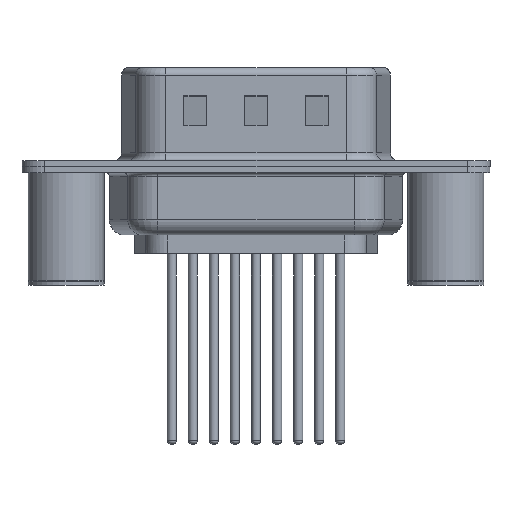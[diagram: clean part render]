
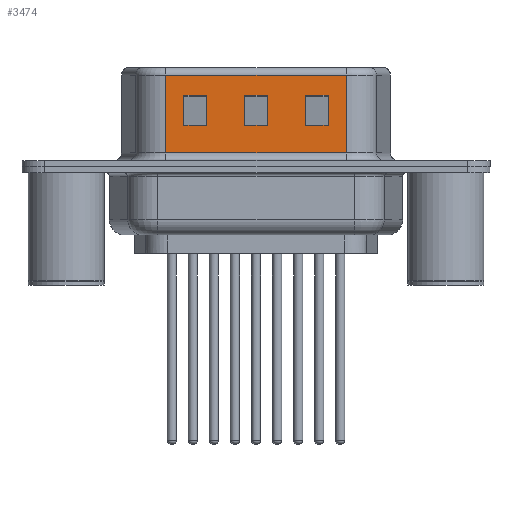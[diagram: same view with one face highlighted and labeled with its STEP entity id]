
A CAD part, front view. The second image highlights one B-rep face of the part: STEP entity #3474.
In plain terms, the highlighted planar face has unit normal (0, -1, 0).
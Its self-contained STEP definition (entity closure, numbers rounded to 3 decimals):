
#218 = CARTESIAN_POINT ( 'NONE',  ( 7.75, -4.55, 2.705 ) ) ;
#254 = CARTESIAN_POINT ( 'NONE',  ( 14.451, -4.55, 2.705 ) ) ;
#311 = DIRECTION ( 'NONE',  ( -1., 0., 0. ) ) ;
#480 = CARTESIAN_POINT ( 'NONE',  ( 22.451, -4.55, 2.705 ) ) ;
#491 = CARTESIAN_POINT ( 'NONE',  ( 11.75, -4.55, 6.52 ) ) ;
#503 = CARTESIAN_POINT ( 'NONE',  ( 18.451, -4.55, 0.9 ) ) ;
#578 = CARTESIAN_POINT ( 'NONE',  ( 9.25, -4.55, 4.705 ) ) ;
#632 = CARTESIAN_POINT ( 'NONE',  ( 6.549, -4.55, 6.02 ) ) ;
#977 = VERTEX_POINT ( 'NONE', #578 ) ;
#1169 = CARTESIAN_POINT ( 'NONE',  ( 18.451, -4.55, 4.705 ) ) ;
#1282 = VERTEX_POINT ( 'NONE', #12414 ) ;
#1305 = LINE ( 'NONE', #480, #1506 ) ;
#1433 = CARTESIAN_POINT ( 'NONE',  ( 17.25, -4.55, 2.705 ) ) ;
#1506 = VECTOR ( 'NONE', #10874, 1000. ) ;
#1622 = EDGE_CURVE ( 'NONE', #1282, #977, #7568, .T. ) ;
#1678 = VERTEX_POINT ( 'NONE', #4030 ) ;
#1951 = CARTESIAN_POINT ( 'NONE',  ( 14.451, -4.55, 4.705 ) ) ;
#2179 = ORIENTED_EDGE ( 'NONE', *, *, #2332, .F. ) ;
#2308 = DIRECTION ( 'NONE',  ( 0., 0., 1. ) ) ;
#2332 = EDGE_CURVE ( 'NONE', #5560, #8779, #4738, .T. ) ;
#2356 = EDGE_CURVE ( 'NONE', #13683, #6903, #7967, .T. ) ;
#2851 = CARTESIAN_POINT ( 'NONE',  ( 15.75, -4.55, 6.52 ) ) ;
#2897 = VERTEX_POINT ( 'NONE', #1433 ) ;
#3019 = CARTESIAN_POINT ( 'NONE',  ( 7.75, -4.55, 6.52 ) ) ;
#3036 = ORIENTED_EDGE ( 'NONE', *, *, #8188, .T. ) ;
#3043 = VERTEX_POINT ( 'NONE', #6137 ) ;
#3084 = DIRECTION ( 'NONE',  ( 0., 0., -1. ) ) ;
#3296 = CARTESIAN_POINT ( 'NONE',  ( 18.451, -4.55, 0.9 ) ) ;
#3410 = ORIENTED_EDGE ( 'NONE', *, *, #10835, .T. ) ;
#3474 = ADVANCED_FACE ( 'NONE', ( #7846, #12487, #13536, #14818 ), #11289, .F. ) ;
#3587 = DIRECTION ( 'NONE',  ( 0., 0., -1. ) ) ;
#3903 = VECTOR ( 'NONE', #8540, 1000. ) ;
#4028 = VECTOR ( 'NONE', #6989, 1000. ) ;
#4030 = CARTESIAN_POINT ( 'NONE',  ( 6.549, -4.55, 0.9 ) ) ;
#4054 = EDGE_CURVE ( 'NONE', #2897, #3043, #1305, .T. ) ;
#4115 = CARTESIAN_POINT ( 'NONE',  ( 9.25, -4.55, 6.52 ) ) ;
#4258 = LINE ( 'NONE', #3296, #7991 ) ;
#4315 = VERTEX_POINT ( 'NONE', #9978 ) ;
#4575 = EDGE_CURVE ( 'NONE', #14116, #4315, #5269, .T. ) ;
#4643 = EDGE_CURVE ( 'NONE', #6903, #1282, #14329, .T. ) ;
#4707 = CARTESIAN_POINT ( 'NONE',  ( 17.25, -4.55, 6.52 ) ) ;
#4738 = LINE ( 'NONE', #6979, #11361 ) ;
#4763 = ORIENTED_EDGE ( 'NONE', *, *, #12984, .T. ) ;
#4870 = DIRECTION ( 'NONE',  ( 1., 0., 0. ) ) ;
#4931 = CARTESIAN_POINT ( 'NONE',  ( 18.451, -4.55, 6.02 ) ) ;
#4947 = LINE ( 'NONE', #6851, #12132 ) ;
#4975 = LINE ( 'NONE', #491, #10548 ) ;
#5015 = EDGE_LOOP ( 'NONE', ( #3036, #10046, #6548, #5702 ) ) ;
#5024 = EDGE_CURVE ( 'NONE', #3043, #6532, #7494, .T. ) ;
#5044 = VECTOR ( 'NONE', #3084, 1000. ) ;
#5077 = EDGE_CURVE ( 'NONE', #4315, #6470, #13031, .T. ) ;
#5103 = VECTOR ( 'NONE', #6162, 1000. ) ;
#5244 = CARTESIAN_POINT ( 'NONE',  ( 11.75, -4.55, 2.705 ) ) ;
#5247 = CARTESIAN_POINT ( 'NONE',  ( 18.451, -4.55, 2.705 ) ) ;
#5269 = LINE ( 'NONE', #10876, #7737 ) ;
#5286 = VECTOR ( 'NONE', #9159, 1000. ) ;
#5560 = VERTEX_POINT ( 'NONE', #4931 ) ;
#5702 = ORIENTED_EDGE ( 'NONE', *, *, #9033, .T. ) ;
#5853 = LINE ( 'NONE', #8173, #14726 ) ;
#6130 = EDGE_LOOP ( 'NONE', ( #2179, #13616, #13368, #8564 ) ) ;
#6137 = CARTESIAN_POINT ( 'NONE',  ( 15.75, -4.55, 2.705 ) ) ;
#6162 = DIRECTION ( 'NONE',  ( 0., 0., 1. ) ) ;
#6470 = VERTEX_POINT ( 'NONE', #5244 ) ;
#6532 = VERTEX_POINT ( 'NONE', #7413 ) ;
#6548 = ORIENTED_EDGE ( 'NONE', *, *, #5024, .T. ) ;
#6584 = VECTOR ( 'NONE', #12469, 1000. ) ;
#6648 = EDGE_CURVE ( 'NONE', #1678, #8779, #4258, .T. ) ;
#6851 = CARTESIAN_POINT ( 'NONE',  ( 22.451, -4.55, 4.705 ) ) ;
#6903 = VERTEX_POINT ( 'NONE', #218 ) ;
#6979 = CARTESIAN_POINT ( 'NONE',  ( 18.451, -4.55, 6.52 ) ) ;
#6989 = DIRECTION ( 'NONE',  ( 1., 0., 0. ) ) ;
#7223 = VECTOR ( 'NONE', #9804, 1000. ) ;
#7413 = CARTESIAN_POINT ( 'NONE',  ( 15.75, -4.55, 4.705 ) ) ;
#7473 = ORIENTED_EDGE ( 'NONE', *, *, #4643, .T. ) ;
#7494 = LINE ( 'NONE', #2851, #8460 ) ;
#7542 = CARTESIAN_POINT ( 'NONE',  ( 11.75, -4.55, 4.705 ) ) ;
#7568 = LINE ( 'NONE', #1951, #7223 ) ;
#7737 = VECTOR ( 'NONE', #8709, 1000. ) ;
#7845 = EDGE_CURVE ( 'NONE', #5560, #10954, #5853, .T. ) ;
#7846 = FACE_BOUND ( 'NONE', #14136, .T. ) ;
#7905 = LINE ( 'NONE', #1169, #4028 ) ;
#7967 = LINE ( 'NONE', #254, #6584 ) ;
#7991 = VECTOR ( 'NONE', #8911, 1000. ) ;
#8173 = CARTESIAN_POINT ( 'NONE',  ( 18.451, -4.55, 6.02 ) ) ;
#8188 = EDGE_CURVE ( 'NONE', #12977, #2897, #11604, .T. ) ;
#8460 = VECTOR ( 'NONE', #10931, 1000. ) ;
#8540 = DIRECTION ( 'NONE',  ( -1., 0., 0. ) ) ;
#8564 = ORIENTED_EDGE ( 'NONE', *, *, #6648, .T. ) ;
#8709 = DIRECTION ( 'NONE',  ( 0., 0., -1. ) ) ;
#8731 = ORIENTED_EDGE ( 'NONE', *, *, #2356, .T. ) ;
#8779 = VERTEX_POINT ( 'NONE', #503 ) ;
#8911 = DIRECTION ( 'NONE',  ( 1., 0., 0. ) ) ;
#8938 = VERTEX_POINT ( 'NONE', #7542 ) ;
#9033 = EDGE_CURVE ( 'NONE', #6532, #12977, #4947, .T. ) ;
#9159 = DIRECTION ( 'NONE',  ( 0., 0., -1. ) ) ;
#9163 = ORIENTED_EDGE ( 'NONE', *, *, #4575, .T. ) ;
#9224 = VECTOR ( 'NONE', #3587, 1000. ) ;
#9248 = ORIENTED_EDGE ( 'NONE', *, *, #1622, .T. ) ;
#9375 = EDGE_LOOP ( 'NONE', ( #3410, #9163, #9984, #11782 ) ) ;
#9768 = CARTESIAN_POINT ( 'NONE',  ( 9.25, -4.55, 2.705 ) ) ;
#9804 = DIRECTION ( 'NONE',  ( 1., 0., 0. ) ) ;
#9978 = CARTESIAN_POINT ( 'NONE',  ( 13.25, -4.55, 2.705 ) ) ;
#9984 = ORIENTED_EDGE ( 'NONE', *, *, #5077, .T. ) ;
#10046 = ORIENTED_EDGE ( 'NONE', *, *, #4054, .T. ) ;
#10548 = VECTOR ( 'NONE', #10737, 1000. ) ;
#10737 = DIRECTION ( 'NONE',  ( 0., 0., 1. ) ) ;
#10835 = EDGE_CURVE ( 'NONE', #8938, #14116, #7905, .T. ) ;
#10874 = DIRECTION ( 'NONE',  ( -1., 0., 0. ) ) ;
#10876 = CARTESIAN_POINT ( 'NONE',  ( 13.25, -4.55, 6.52 ) ) ;
#10931 = DIRECTION ( 'NONE',  ( 0., 0., 1. ) ) ;
#10954 = VERTEX_POINT ( 'NONE', #632 ) ;
#11289 = PLANE ( 'NONE',  #13202 ) ;
#11361 = VECTOR ( 'NONE', #11556, 1000. ) ;
#11556 = DIRECTION ( 'NONE',  ( 0., 0., -1. ) ) ;
#11604 = LINE ( 'NONE', #4707, #9224 ) ;
#11782 = ORIENTED_EDGE ( 'NONE', *, *, #13592, .T. ) ;
#12132 = VECTOR ( 'NONE', #4870, 1000. ) ;
#12288 = CARTESIAN_POINT ( 'NONE',  ( 17.25, -4.55, 4.705 ) ) ;
#12414 = CARTESIAN_POINT ( 'NONE',  ( 7.75, -4.55, 4.705 ) ) ;
#12416 = DIRECTION ( 'NONE',  ( 0., 1., 0. ) ) ;
#12469 = DIRECTION ( 'NONE',  ( -1., 0., 0. ) ) ;
#12487 = FACE_BOUND ( 'NONE', #5015, .T. ) ;
#12558 = CARTESIAN_POINT ( 'NONE',  ( 18.451, -4.55, 6.52 ) ) ;
#12606 = EDGE_CURVE ( 'NONE', #10954, #1678, #14787, .T. ) ;
#12977 = VERTEX_POINT ( 'NONE', #12288 ) ;
#12984 = EDGE_CURVE ( 'NONE', #977, #13683, #13337, .T. ) ;
#13031 = LINE ( 'NONE', #5247, #3903 ) ;
#13202 = AXIS2_PLACEMENT_3D ( 'NONE', #12558, #12416, #2308 ) ;
#13337 = LINE ( 'NONE', #4115, #5044 ) ;
#13368 = ORIENTED_EDGE ( 'NONE', *, *, #12606, .T. ) ;
#13536 = FACE_BOUND ( 'NONE', #9375, .T. ) ;
#13592 = EDGE_CURVE ( 'NONE', #6470, #8938, #4975, .T. ) ;
#13616 = ORIENTED_EDGE ( 'NONE', *, *, #7845, .T. ) ;
#13683 = VERTEX_POINT ( 'NONE', #9768 ) ;
#13798 = CARTESIAN_POINT ( 'NONE',  ( 6.549, -4.55, 6.52 ) ) ;
#14116 = VERTEX_POINT ( 'NONE', #14249 ) ;
#14136 = EDGE_LOOP ( 'NONE', ( #4763, #8731, #7473, #9248 ) ) ;
#14249 = CARTESIAN_POINT ( 'NONE',  ( 13.25, -4.55, 4.705 ) ) ;
#14329 = LINE ( 'NONE', #3019, #5103 ) ;
#14726 = VECTOR ( 'NONE', #311, 1000. ) ;
#14787 = LINE ( 'NONE', #13798, #5286 ) ;
#14818 = FACE_OUTER_BOUND ( 'NONE', #6130, .T. ) ;
